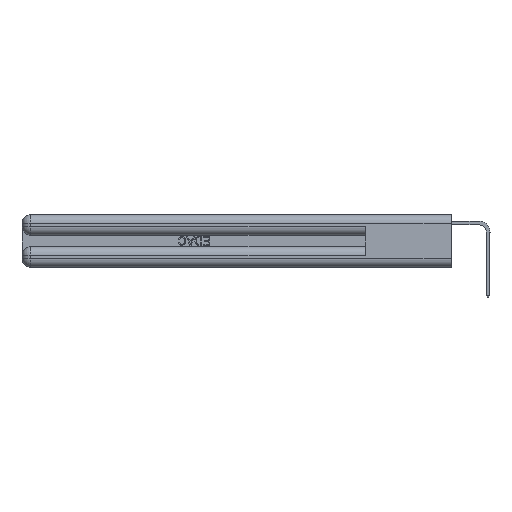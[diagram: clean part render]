
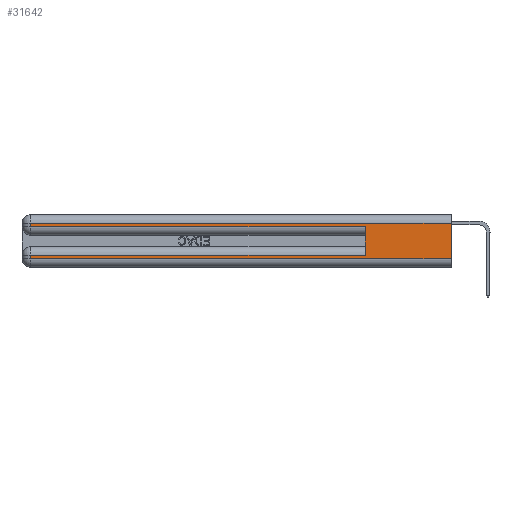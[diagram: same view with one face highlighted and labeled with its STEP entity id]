
A CAD part, left-side view. The second image highlights one B-rep face of the part: STEP entity #31642.
In plain terms, the highlighted planar face has unit normal (-1, 0, 0).
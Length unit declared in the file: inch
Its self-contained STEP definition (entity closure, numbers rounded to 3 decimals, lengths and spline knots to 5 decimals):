
#464 = CARTESIAN_POINT ( 'NONE',  ( 0., 0., 0.06 ) ) ;
#950 = LINE ( 'NONE', #9886, #2592 ) ;
#1270 = DIRECTION ( 'NONE',  ( 0., 1., 0. ) ) ;
#1430 = CARTESIAN_POINT ( 'NONE',  ( 0., 0.6, 0.085 ) ) ;
#1760 = VERTEX_POINT ( 'NONE', #5101 ) ;
#2160 = CARTESIAN_POINT ( 'NONE',  ( 0., 0., 0.37 ) ) ;
#2592 = VECTOR ( 'NONE', #25364, 39.37008 ) ;
#5054 = AXIS2_PLACEMENT_3D ( 'NONE', #30569, #28117, #12775 ) ;
#5101 = CARTESIAN_POINT ( 'NONE',  ( 0., 0.6, 0.285 ) ) ;
#5187 = EDGE_CURVE ( 'NONE', #11789, #16656, #33122, .T. ) ;
#5755 = ORIENTED_EDGE ( 'NONE', *, *, #10057, .T. ) ;
#5875 = CARTESIAN_POINT ( 'NONE',  ( 0., 2.94, 0.085 ) ) ;
#6032 = VECTOR ( 'NONE', #23834, 39.37008 ) ;
#6328 = VECTOR ( 'NONE', #18078, 39.37008 ) ;
#6612 = CARTESIAN_POINT ( 'NONE',  ( 0., 0., 0.085 ) ) ;
#6658 = CARTESIAN_POINT ( 'NONE',  ( 0., 0., 0.06 ) ) ;
#7767 = CARTESIAN_POINT ( 'NONE',  ( 0., 0., 0.285 ) ) ;
#7834 = VECTOR ( 'NONE', #9949, 39.37008 ) ;
#9224 = VECTOR ( 'NONE', #30872, 39.37008 ) ;
#9296 = VERTEX_POINT ( 'NONE', #13618 ) ;
#9441 = LINE ( 'NONE', #2160, #7834 ) ;
#9886 = CARTESIAN_POINT ( 'NONE',  ( 0., 2.94, 0.37 ) ) ;
#9945 = FACE_OUTER_BOUND ( 'NONE', #14683, .T. ) ;
#9949 = DIRECTION ( 'NONE',  ( 0., 0., -1. ) ) ;
#10057 = EDGE_CURVE ( 'NONE', #23709, #9296, #29995, .T. ) ;
#10487 = ORIENTED_EDGE ( 'NONE', *, *, #14787, .T. ) ;
#11789 = VERTEX_POINT ( 'NONE', #14761 ) ;
#11790 = DIRECTION ( 'NONE',  ( 0., 1., 0. ) ) ;
#12603 = VERTEX_POINT ( 'NONE', #5875 ) ;
#12704 = VECTOR ( 'NONE', #15733, 39.37008 ) ;
#12775 = DIRECTION ( 'NONE',  ( 0., 0., -1. ) ) ;
#12830 = VERTEX_POINT ( 'NONE', #1430 ) ;
#12965 = CARTESIAN_POINT ( 'NONE',  ( 0., 2.94, 0.37 ) ) ;
#13618 = CARTESIAN_POINT ( 'NONE',  ( 0., 2.94, 0.31 ) ) ;
#13792 = ORIENTED_EDGE ( 'NONE', *, *, #17340, .T. ) ;
#13946 = LINE ( 'NONE', #7767, #6328 ) ;
#14000 = ORIENTED_EDGE ( 'NONE', *, *, #21339, .F. ) ;
#14683 = EDGE_LOOP ( 'NONE', ( #21043, #5755, #10487, #30431, #14000, #18287, #13792, #19523 ) ) ;
#14761 = CARTESIAN_POINT ( 'NONE',  ( 0., 2.94, 0.06 ) ) ;
#14787 = EDGE_CURVE ( 'NONE', #9296, #24926, #28087, .T. ) ;
#15413 = VECTOR ( 'NONE', #11790, 39.37008 ) ;
#15632 = CARTESIAN_POINT ( 'NONE',  ( 0., 0., 0.31 ) ) ;
#15733 = DIRECTION ( 'NONE',  ( 0., -1., 0. ) ) ;
#16030 = CARTESIAN_POINT ( 'NONE',  ( 0., 0.6, 0.145 ) ) ;
#16656 = VERTEX_POINT ( 'NONE', #6658 ) ;
#16667 = CARTESIAN_POINT ( 'NONE',  ( 0., 0., 0.31 ) ) ;
#17294 = EDGE_CURVE ( 'NONE', #12830, #12603, #23090, .T. ) ;
#17340 = EDGE_CURVE ( 'NONE', #12603, #11789, #950, .T. ) ;
#18078 = DIRECTION ( 'NONE',  ( 0., -1., 0. ) ) ;
#18287 = ORIENTED_EDGE ( 'NONE', *, *, #17294, .T. ) ;
#19523 = ORIENTED_EDGE ( 'NONE', *, *, #5187, .T. ) ;
#20360 = PLANE ( 'NONE',  #5054 ) ;
#21043 = ORIENTED_EDGE ( 'NONE', *, *, #24221, .F. ) ;
#21339 = EDGE_CURVE ( 'NONE', #12830, #1760, #26502, .T. ) ;
#23090 = LINE ( 'NONE', #6612, #15413 ) ;
#23709 = VERTEX_POINT ( 'NONE', #15632 ) ;
#23834 = DIRECTION ( 'NONE',  ( 0., 0., 1. ) ) ;
#24221 = EDGE_CURVE ( 'NONE', #23709, #16656, #9441, .T. ) ;
#24810 = VECTOR ( 'NONE', #1270, 39.37008 ) ;
#24926 = VERTEX_POINT ( 'NONE', #28178 ) ;
#25364 = DIRECTION ( 'NONE',  ( 0., 0., -1. ) ) ;
#26502 = LINE ( 'NONE', #16030, #6032 ) ;
#28087 = LINE ( 'NONE', #12965, #9224 ) ;
#28117 = DIRECTION ( 'NONE',  ( 1., 0., 0. ) ) ;
#28178 = CARTESIAN_POINT ( 'NONE',  ( 0., 2.94, 0.285 ) ) ;
#29995 = LINE ( 'NONE', #16667, #24810 ) ;
#30431 = ORIENTED_EDGE ( 'NONE', *, *, #32230, .T. ) ;
#30569 = CARTESIAN_POINT ( 'NONE',  ( 0., 0., 0.37 ) ) ;
#30872 = DIRECTION ( 'NONE',  ( 0., 0., -1. ) ) ;
#31642 = ADVANCED_FACE ( 'NONE', ( #9945 ), #20360, .F. ) ;
#32230 = EDGE_CURVE ( 'NONE', #24926, #1760, #13946, .T. ) ;
#33122 = LINE ( 'NONE', #464, #12704 ) ;
